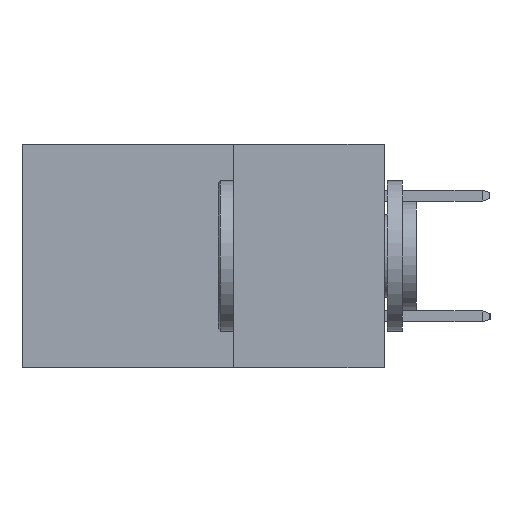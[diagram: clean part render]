
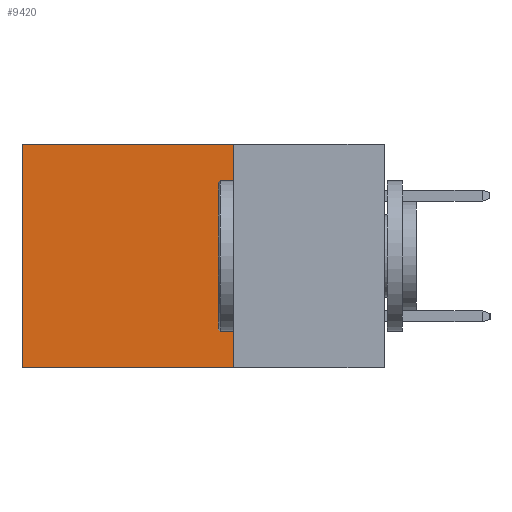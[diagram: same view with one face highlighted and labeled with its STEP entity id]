
A CAD part, left-side view. The second image highlights one B-rep face of the part: STEP entity #9420.
In plain terms, the highlighted planar face has unit normal (-1, 0, 0).
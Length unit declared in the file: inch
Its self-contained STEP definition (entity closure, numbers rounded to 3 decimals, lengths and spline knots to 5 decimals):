
#81 = EDGE_CURVE ( 'NONE', #8591, #10072, #3233, .T. ) ;
#551 = VECTOR ( 'NONE', #2353, 39.37008 ) ;
#792 = CARTESIAN_POINT ( 'NONE',  ( 0.2615, 0.25, -0.37 ) ) ;
#831 = CARTESIAN_POINT ( 'NONE',  ( 0.2615, 0.6, -0.37 ) ) ;
#1070 = LINE ( 'NONE', #6311, #551 ) ;
#1285 = EDGE_CURVE ( 'NONE', #8813, #10072, #6694, .T. ) ;
#1384 = DIRECTION ( 'NONE',  ( 0., 1., 0. ) ) ;
#2242 = DIRECTION ( 'NONE',  ( 0., 1., 0. ) ) ;
#2353 = DIRECTION ( 'NONE',  ( 0., 0., -1. ) ) ;
#2698 = EDGE_LOOP ( 'NONE', ( #9912, #3895, #5456, #7394 ) ) ;
#2738 = VECTOR ( 'NONE', #1384, 39.37008 ) ;
#2932 = CARTESIAN_POINT ( 'NONE',  ( 0.2615, 0.6, -0.37 ) ) ;
#3233 = LINE ( 'NONE', #2932, #6699 ) ;
#3383 = DIRECTION ( 'NONE',  ( 0., 0., -1. ) ) ;
#3895 = ORIENTED_EDGE ( 'NONE', *, *, #1285, .F. ) ;
#3950 = DIRECTION ( 'NONE',  ( 0., 0., -1. ) ) ;
#4682 = VERTEX_POINT ( 'NONE', #7015 ) ;
#5065 = LINE ( 'NONE', #7793, #2738 ) ;
#5209 = FACE_OUTER_BOUND ( 'NONE', #2698, .T. ) ;
#5314 = AXIS2_PLACEMENT_3D ( 'NONE', #6518, #8131, #3383 ) ;
#5456 = ORIENTED_EDGE ( 'NONE', *, *, #6051, .F. ) ;
#6051 = EDGE_CURVE ( 'NONE', #4682, #8813, #1070, .T. ) ;
#6311 = CARTESIAN_POINT ( 'NONE',  ( 0.2615, 0.25, -0.37 ) ) ;
#6503 = EDGE_CURVE ( 'NONE', #4682, #8591, #5065, .T. ) ;
#6518 = CARTESIAN_POINT ( 'NONE',  ( 0.2615, 0.25, -0.37 ) ) ;
#6694 = LINE ( 'NONE', #792, #8543 ) ;
#6699 = VECTOR ( 'NONE', #3950, 39.37008 ) ;
#7015 = CARTESIAN_POINT ( 'NONE',  ( 0.2615, 0.25, 0. ) ) ;
#7358 = PLANE ( 'NONE',  #5314 ) ;
#7394 = ORIENTED_EDGE ( 'NONE', *, *, #6503, .T. ) ;
#7793 = CARTESIAN_POINT ( 'NONE',  ( 0.2615, 0.25, 0. ) ) ;
#8131 = DIRECTION ( 'NONE',  ( 1., 0., 0. ) ) ;
#8215 = CARTESIAN_POINT ( 'NONE',  ( 0.2615, 0.25, -0.37 ) ) ;
#8543 = VECTOR ( 'NONE', #2242, 39.37008 ) ;
#8591 = VERTEX_POINT ( 'NONE', #10180 ) ;
#8813 = VERTEX_POINT ( 'NONE', #8215 ) ;
#9420 = ADVANCED_FACE ( 'NONE', ( #5209 ), #7358, .F. ) ;
#9912 = ORIENTED_EDGE ( 'NONE', *, *, #81, .T. ) ;
#10072 = VERTEX_POINT ( 'NONE', #831 ) ;
#10180 = CARTESIAN_POINT ( 'NONE',  ( 0.2615, 0.6, 0. ) ) ;
